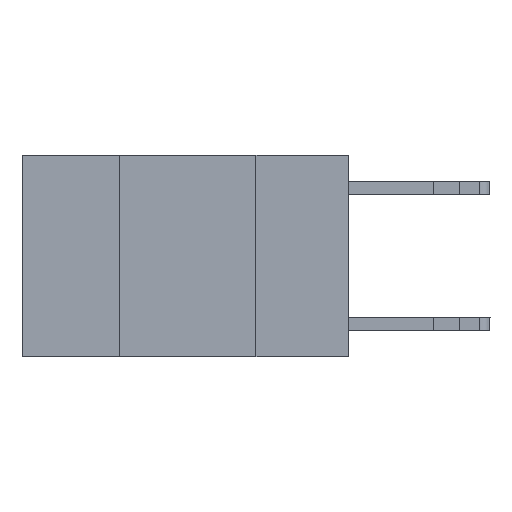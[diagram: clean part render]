
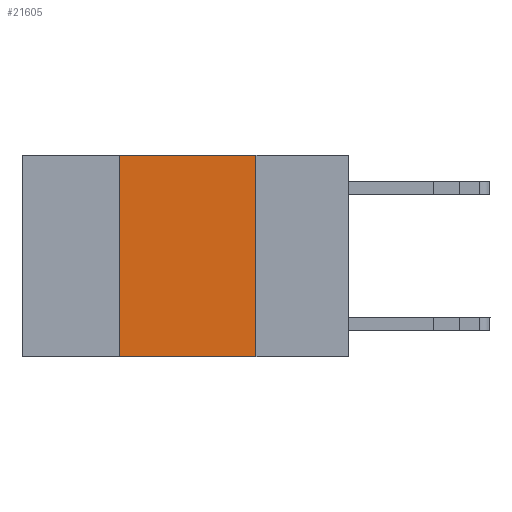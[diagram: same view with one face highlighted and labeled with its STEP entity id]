
A CAD part, left-side view. The second image highlights one B-rep face of the part: STEP entity #21605.
In plain terms, the highlighted planar face has unit normal (-1, 0, 0).
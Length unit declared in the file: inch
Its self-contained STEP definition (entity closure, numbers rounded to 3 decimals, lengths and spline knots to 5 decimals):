
#744 = CARTESIAN_POINT ( 'NONE',  ( 0., 0.17, 0. ) ) ;
#1440 = VERTEX_POINT ( 'NONE', #10256 ) ;
#2784 = VERTEX_POINT ( 'NONE', #7478 ) ;
#3724 = PLANE ( 'NONE',  #13463 ) ;
#4913 = CARTESIAN_POINT ( 'NONE',  ( 0., 0.6, -0.37 ) ) ;
#5038 = EDGE_CURVE ( 'NONE', #12843, #16845, #20548, .T. ) ;
#5767 = VECTOR ( 'NONE', #10981, 39.37008 ) ;
#5892 = LINE ( 'NONE', #18919, #5767 ) ;
#7478 = CARTESIAN_POINT ( 'NONE',  ( 0., 0.42, 0. ) ) ;
#7972 = DIRECTION ( 'NONE',  ( 0., 0., -1. ) ) ;
#9260 = EDGE_LOOP ( 'NONE', ( #9765, #10131, #10237, #10469 ) ) ;
#9576 = DIRECTION ( 'NONE',  ( 0., 0., -1. ) ) ;
#9700 = CARTESIAN_POINT ( 'NONE',  ( 0., 0.17, 0. ) ) ;
#9765 = ORIENTED_EDGE ( 'NONE', *, *, #5038, .F. ) ;
#10131 = ORIENTED_EDGE ( 'NONE', *, *, #18225, .F. ) ;
#10237 = ORIENTED_EDGE ( 'NONE', *, *, #23248, .F. ) ;
#10256 = CARTESIAN_POINT ( 'NONE',  ( 0., 0.42, -0.37 ) ) ;
#10469 = ORIENTED_EDGE ( 'NONE', *, *, #19280, .T. ) ;
#10981 = DIRECTION ( 'NONE',  ( 0., 0., 1. ) ) ;
#11026 = LINE ( 'NONE', #4913, #11192 ) ;
#11189 = FACE_OUTER_BOUND ( 'NONE', #9260, .T. ) ;
#11192 = VECTOR ( 'NONE', #17253, 39.37008 ) ;
#12843 = VERTEX_POINT ( 'NONE', #744 ) ;
#13463 = AXIS2_PLACEMENT_3D ( 'NONE', #18145, #20103, #7972 ) ;
#15260 = CARTESIAN_POINT ( 'NONE',  ( 0., 0.17, -0.37 ) ) ;
#16845 = VERTEX_POINT ( 'NONE', #15260 ) ;
#17253 = DIRECTION ( 'NONE',  ( 0., -1., 0. ) ) ;
#18145 = CARTESIAN_POINT ( 'NONE',  ( 0., 0.6, 0. ) ) ;
#18225 = EDGE_CURVE ( 'NONE', #2784, #12843, #20484, .T. ) ;
#18919 = CARTESIAN_POINT ( 'NONE',  ( 0., 0.42, 0. ) ) ;
#19280 = EDGE_CURVE ( 'NONE', #1440, #16845, #11026, .T. ) ;
#19498 = VECTOR ( 'NONE', #9576, 39.37008 ) ;
#20103 = DIRECTION ( 'NONE',  ( 1., 0., 0. ) ) ;
#20457 = VECTOR ( 'NONE', #24054, 39.37008 ) ;
#20484 = LINE ( 'NONE', #22020, #20457 ) ;
#20548 = LINE ( 'NONE', #9700, #19498 ) ;
#21605 = ADVANCED_FACE ( 'NONE', ( #11189 ), #3724, .F. ) ;
#22020 = CARTESIAN_POINT ( 'NONE',  ( 0., 0.6, 0. ) ) ;
#23248 = EDGE_CURVE ( 'NONE', #1440, #2784, #5892, .T. ) ;
#24054 = DIRECTION ( 'NONE',  ( 0., -1., 0. ) ) ;
